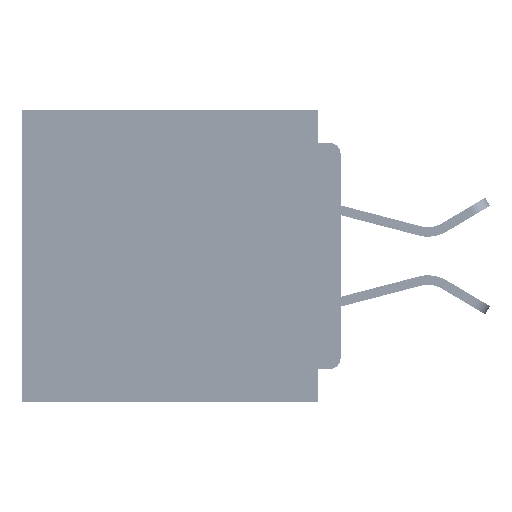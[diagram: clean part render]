
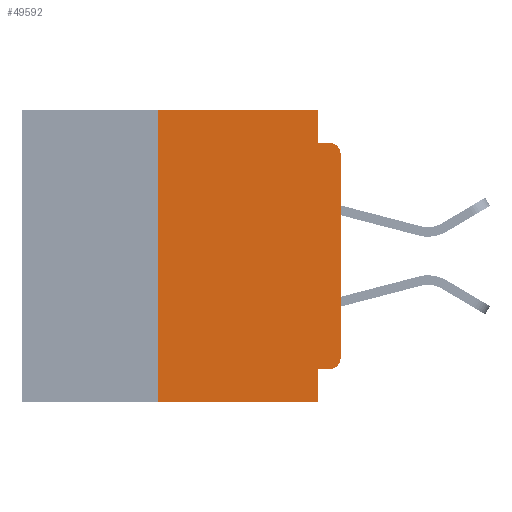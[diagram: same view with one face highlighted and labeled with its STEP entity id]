
A CAD part, left-side view. The second image highlights one B-rep face of the part: STEP entity #49592.
In plain terms, the highlighted planar face has unit normal (-1, 0, 0).
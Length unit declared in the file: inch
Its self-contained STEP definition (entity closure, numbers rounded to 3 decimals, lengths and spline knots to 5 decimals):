
#445 = AXIS2_PLACEMENT_3D ( 'NONE', #15095, #45032, #19443 ) ;
#1072 = CARTESIAN_POINT ( 'NONE',  ( 0., 0.437, 0. ) ) ;
#1384 = DIRECTION ( 'NONE',  ( 0., 0., 1. ) ) ;
#1402 = ORIENTED_EDGE ( 'NONE', *, *, #20028, .T. ) ;
#1413 = VECTOR ( 'NONE', #1438, 39.37008 ) ;
#1438 = DIRECTION ( 'NONE',  ( 0., -1., 0. ) ) ;
#3546 = CARTESIAN_POINT ( 'NONE',  ( 0., 0.031, -0.045 ) ) ;
#4272 = LINE ( 'NONE', #39774, #48568 ) ;
#5527 = DIRECTION ( 'NONE',  ( 0., 0., -1. ) ) ;
#6308 = LINE ( 'NONE', #34642, #50588 ) ;
#9434 = CARTESIAN_POINT ( 'NONE',  ( 0., 0.25, -0.4 ) ) ;
#9754 = DIRECTION ( 'NONE',  ( 0., 0., -1. ) ) ;
#9792 = VECTOR ( 'NONE', #1384, 39.37008 ) ;
#9994 = EDGE_CURVE ( 'NONE', #47650, #15308, #43180, .T. ) ;
#12039 = LINE ( 'NONE', #29780, #33546 ) ;
#12959 = CARTESIAN_POINT ( 'NONE',  ( 0., 0.25, -0.4 ) ) ;
#13101 = AXIS2_PLACEMENT_3D ( 'NONE', #45340, #19757, #49614 ) ;
#13683 = CIRCLE ( 'NONE', #13101, 0.015 ) ;
#14159 = CARTESIAN_POINT ( 'NONE',  ( 0., 0.25, 0. ) ) ;
#15095 = CARTESIAN_POINT ( 'NONE',  ( 0., 0.015, -0.34 ) ) ;
#15118 = EDGE_CURVE ( 'NONE', #20221, #16924, #13683, .T. ) ;
#15257 = VERTEX_POINT ( 'NONE', #46448 ) ;
#15308 = VERTEX_POINT ( 'NONE', #33986 ) ;
#15389 = VECTOR ( 'NONE', #38653, 39.37008 ) ;
#16924 = VERTEX_POINT ( 'NONE', #45163 ) ;
#17232 = CIRCLE ( 'NONE', #445, 0.015 ) ;
#17435 = VECTOR ( 'NONE', #36860, 39.37008 ) ;
#19443 = DIRECTION ( 'NONE',  ( 0., 0., -1. ) ) ;
#19757 = DIRECTION ( 'NONE',  ( -1., 0., 0. ) ) ;
#19907 = ORIENTED_EDGE ( 'NONE', *, *, #47065, .T. ) ;
#20028 = EDGE_CURVE ( 'NONE', #32127, #20221, #34035, .T. ) ;
#20107 = EDGE_CURVE ( 'NONE', #15257, #32127, #17232, .T. ) ;
#20221 = VERTEX_POINT ( 'NONE', #51044 ) ;
#21084 = EDGE_CURVE ( 'NONE', #15308, #27599, #4272, .T. ) ;
#21997 = CARTESIAN_POINT ( 'NONE',  ( 0., 0.437, 0. ) ) ;
#22763 = AXIS2_PLACEMENT_3D ( 'NONE', #1072, #31345, #5527 ) ;
#23511 = ORIENTED_EDGE ( 'NONE', *, *, #50422, .F. ) ;
#26864 = LINE ( 'NONE', #12959, #15389 ) ;
#27054 = PLANE ( 'NONE',  #22763 ) ;
#27599 = VERTEX_POINT ( 'NONE', #3546 ) ;
#28021 = VERTEX_POINT ( 'NONE', #36414 ) ;
#28107 = CARTESIAN_POINT ( 'NONE',  ( 0., 0.031, -0.4 ) ) ;
#29543 = ORIENTED_EDGE ( 'NONE', *, *, #21084, .F. ) ;
#29780 = CARTESIAN_POINT ( 'NONE',  ( 0., 0., -0.045 ) ) ;
#31345 = DIRECTION ( 'NONE',  ( 1., 0., 0. ) ) ;
#31776 = VERTEX_POINT ( 'NONE', #9434 ) ;
#32127 = VERTEX_POINT ( 'NONE', #50783 ) ;
#33546 = VECTOR ( 'NONE', #34076, 39.37008 ) ;
#33986 = CARTESIAN_POINT ( 'NONE',  ( 0., 0.031, 0. ) ) ;
#34035 = LINE ( 'NONE', #35922, #9792 ) ;
#34076 = DIRECTION ( 'NONE',  ( 0., -1., 0. ) ) ;
#34133 = ORIENTED_EDGE ( 'NONE', *, *, #15118, .T. ) ;
#34642 = CARTESIAN_POINT ( 'NONE',  ( 0., 0., -0.355 ) ) ;
#34818 = DIRECTION ( 'NONE',  ( 0., 1., 0. ) ) ;
#35076 = ORIENTED_EDGE ( 'NONE', *, *, #9994, .F. ) ;
#35855 = LINE ( 'NONE', #52933, #1413 ) ;
#35922 = CARTESIAN_POINT ( 'NONE',  ( 0., 0., 0. ) ) ;
#36414 = CARTESIAN_POINT ( 'NONE',  ( 0., 0.031, -0.355 ) ) ;
#36860 = DIRECTION ( 'NONE',  ( 0., 0., -1. ) ) ;
#37174 = ORIENTED_EDGE ( 'NONE', *, *, #20107, .T. ) ;
#37650 = FACE_OUTER_BOUND ( 'NONE', #47422, .T. ) ;
#38653 = DIRECTION ( 'NONE',  ( 0., 0., 1. ) ) ;
#39774 = CARTESIAN_POINT ( 'NONE',  ( 0., 0.031, 0. ) ) ;
#41882 = VECTOR ( 'NONE', #43273, 39.37008 ) ;
#42118 = EDGE_CURVE ( 'NONE', #15257, #28021, #6308, .T. ) ;
#42863 = LINE ( 'NONE', #28107, #17435 ) ;
#43180 = LINE ( 'NONE', #21997, #41882 ) ;
#43273 = DIRECTION ( 'NONE',  ( 0., -1., 0. ) ) ;
#43435 = ORIENTED_EDGE ( 'NONE', *, *, #51241, .F. ) ;
#45032 = DIRECTION ( 'NONE',  ( -1., 0., 0. ) ) ;
#45163 = CARTESIAN_POINT ( 'NONE',  ( 0., 0.015, -0.045 ) ) ;
#45340 = CARTESIAN_POINT ( 'NONE',  ( 0., 0.015, -0.06 ) ) ;
#46448 = CARTESIAN_POINT ( 'NONE',  ( 0., 0.015, -0.355 ) ) ;
#46531 = ORIENTED_EDGE ( 'NONE', *, *, #42118, .F. ) ;
#47065 = EDGE_CURVE ( 'NONE', #31776, #52811, #35855, .T. ) ;
#47422 = EDGE_LOOP ( 'NONE', ( #1402, #34133, #52246, #29543, #35076, #43435, #19907, #23511, #46531, #37174 ) ) ;
#47650 = VERTEX_POINT ( 'NONE', #14159 ) ;
#48568 = VECTOR ( 'NONE', #9754, 39.37008 ) ;
#49592 = ADVANCED_FACE ( 'NONE', ( #37650 ), #27054, .F. ) ;
#49614 = DIRECTION ( 'NONE',  ( 0., 0., -1. ) ) ;
#49724 = CARTESIAN_POINT ( 'NONE',  ( 0., 0.031, -0.4 ) ) ;
#50422 = EDGE_CURVE ( 'NONE', #28021, #52811, #42863, .T. ) ;
#50517 = EDGE_CURVE ( 'NONE', #27599, #16924, #12039, .T. ) ;
#50588 = VECTOR ( 'NONE', #34818, 39.37008 ) ;
#50783 = CARTESIAN_POINT ( 'NONE',  ( 0., 0., -0.34 ) ) ;
#51044 = CARTESIAN_POINT ( 'NONE',  ( 0., 0., -0.06 ) ) ;
#51241 = EDGE_CURVE ( 'NONE', #31776, #47650, #26864, .T. ) ;
#52246 = ORIENTED_EDGE ( 'NONE', *, *, #50517, .F. ) ;
#52811 = VERTEX_POINT ( 'NONE', #49724 ) ;
#52933 = CARTESIAN_POINT ( 'NONE',  ( 0., 0.437, -0.4 ) ) ;
